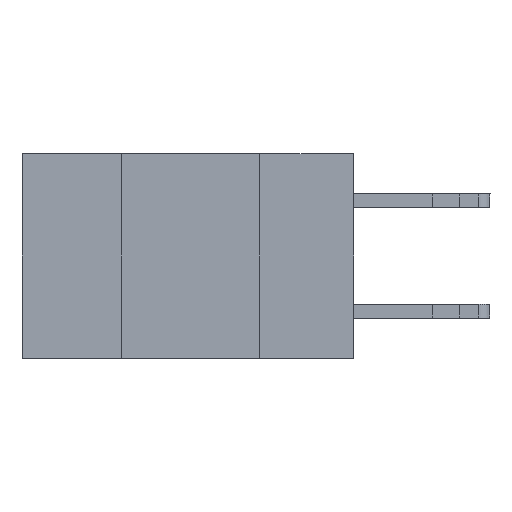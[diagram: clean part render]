
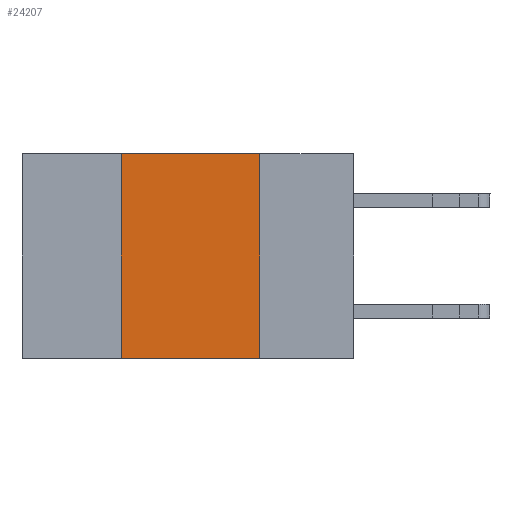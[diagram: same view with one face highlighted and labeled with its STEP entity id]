
A CAD part, left-side view. The second image highlights one B-rep face of the part: STEP entity #24207.
In plain terms, the highlighted planar face has unit normal (-1, 0, 0).
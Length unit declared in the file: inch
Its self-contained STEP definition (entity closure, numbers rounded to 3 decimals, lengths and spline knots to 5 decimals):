
#56 = CARTESIAN_POINT ( 'NONE',  ( 0., 0.6, 0. ) ) ;
#306 = CARTESIAN_POINT ( 'NONE',  ( 0., 0.17, -0.37 ) ) ;
#835 = FACE_OUTER_BOUND ( 'NONE', #13710, .T. ) ;
#2660 = VECTOR ( 'NONE', #20915, 39.37008 ) ;
#3423 = ORIENTED_EDGE ( 'NONE', *, *, #16904, .F. ) ;
#3545 = CARTESIAN_POINT ( 'NONE',  ( 0., 0.17, 0. ) ) ;
#3547 = CARTESIAN_POINT ( 'NONE',  ( 0., 0.42, -0.37 ) ) ;
#4262 = LINE ( 'NONE', #14146, #21039 ) ;
#5292 = DIRECTION ( 'NONE',  ( 0., 0., -1. ) ) ;
#5444 = AXIS2_PLACEMENT_3D ( 'NONE', #24486, #8993, #22970 ) ;
#5619 = VECTOR ( 'NONE', #5292, 39.37008 ) ;
#6189 = VERTEX_POINT ( 'NONE', #3545 ) ;
#6570 = VERTEX_POINT ( 'NONE', #3547 ) ;
#7048 = ORIENTED_EDGE ( 'NONE', *, *, #12045, .F. ) ;
#7390 = EDGE_CURVE ( 'NONE', #6570, #24457, #18180, .T. ) ;
#7613 = VERTEX_POINT ( 'NONE', #19306 ) ;
#8993 = DIRECTION ( 'NONE',  ( 1., 0., 0. ) ) ;
#9868 = EDGE_CURVE ( 'NONE', #6189, #24457, #22368, .T. ) ;
#12045 = EDGE_CURVE ( 'NONE', #6570, #7613, #4262, .T. ) ;
#13085 = CARTESIAN_POINT ( 'NONE',  ( 0., 0.6, -0.37 ) ) ;
#13710 = EDGE_LOOP ( 'NONE', ( #20894, #3423, #7048, #25105 ) ) ;
#14146 = CARTESIAN_POINT ( 'NONE',  ( 0., 0.42, 0. ) ) ;
#16119 = DIRECTION ( 'NONE',  ( 0., 0., 1. ) ) ;
#16904 = EDGE_CURVE ( 'NONE', #7613, #6189, #17363, .T. ) ;
#17363 = LINE ( 'NONE', #56, #24998 ) ;
#18180 = LINE ( 'NONE', #13085, #2660 ) ;
#18592 = PLANE ( 'NONE',  #5444 ) ;
#19306 = CARTESIAN_POINT ( 'NONE',  ( 0., 0.42, 0. ) ) ;
#20757 = CARTESIAN_POINT ( 'NONE',  ( 0., 0.17, 0. ) ) ;
#20894 = ORIENTED_EDGE ( 'NONE', *, *, #9868, .F. ) ;
#20915 = DIRECTION ( 'NONE',  ( 0., -1., 0. ) ) ;
#21039 = VECTOR ( 'NONE', #16119, 39.37008 ) ;
#21269 = DIRECTION ( 'NONE',  ( 0., -1., 0. ) ) ;
#22368 = LINE ( 'NONE', #20757, #5619 ) ;
#22970 = DIRECTION ( 'NONE',  ( 0., 0., -1. ) ) ;
#24207 = ADVANCED_FACE ( 'NONE', ( #835 ), #18592, .F. ) ;
#24457 = VERTEX_POINT ( 'NONE', #306 ) ;
#24486 = CARTESIAN_POINT ( 'NONE',  ( 0., 0.6, 0. ) ) ;
#24998 = VECTOR ( 'NONE', #21269, 39.37008 ) ;
#25105 = ORIENTED_EDGE ( 'NONE', *, *, #7390, .T. ) ;
